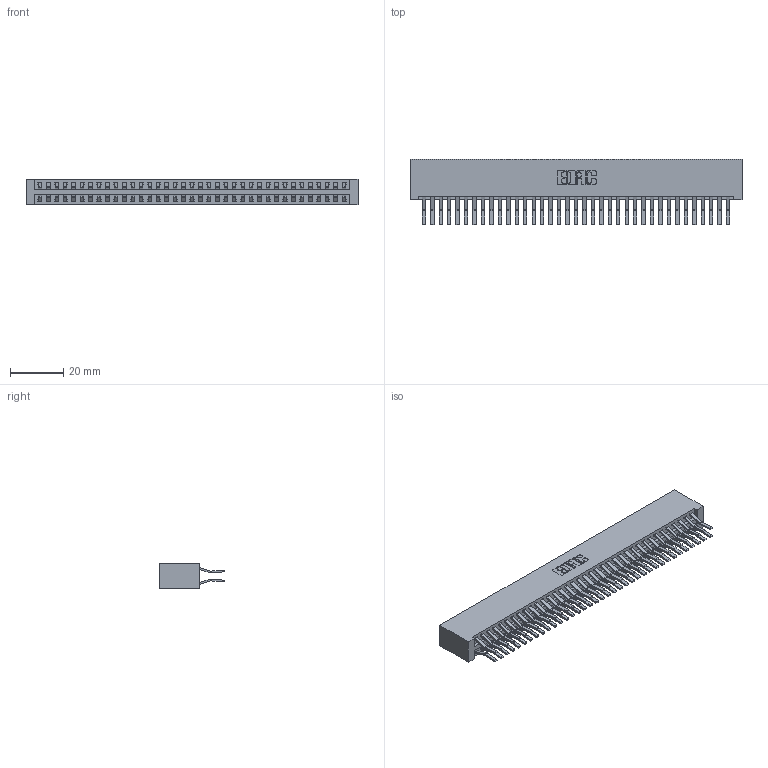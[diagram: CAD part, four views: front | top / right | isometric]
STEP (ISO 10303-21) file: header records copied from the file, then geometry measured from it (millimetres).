
FILE_DESCRIPTION (( 'STEP AP203' ), '1' );
FILE_NAME ('346-074-560-201.STEP', '2018-08-29T03:13:25', ( '' ), ( '' ), 'SwSTEP 2.0', 'SolidWorks 2016', '' );
FILE_SCHEMA (( 'CONFIG_CONTROL_DESIGN' ));
Length unit declared in the file: inch
Products named in the file (3): 346 Part_No Mounting Lugs; 345-292-001_560 Tail; 346-074-560-201
Assembly tree (75 placements, depth 2):
  346-074-560-201
    346 Part_No Mounting Lugs
    345-292-001_560 Tail  x74
Bounding box: 124.71 x 24.78 x 9.4 mm (x, y, z)
Volume: 13180.7 mm3; surface area: 19496.4 mm2
Topology: 75 solids, 75 shells, 4110 faces, 12219 edges, 8046 vertices
Faces by surface type: plane 2662, cylinder 1448
Entity records: 24631 total; most frequent: CARTESIAN_POINT 4064, ORIENTED_EDGE 3998, DIRECTION 3631, EDGE_CURVE 1999, VECTOR 1723, LINE 1723, VERTEX_POINT 1330, AXIS2_PLACEMENT_3D 954
